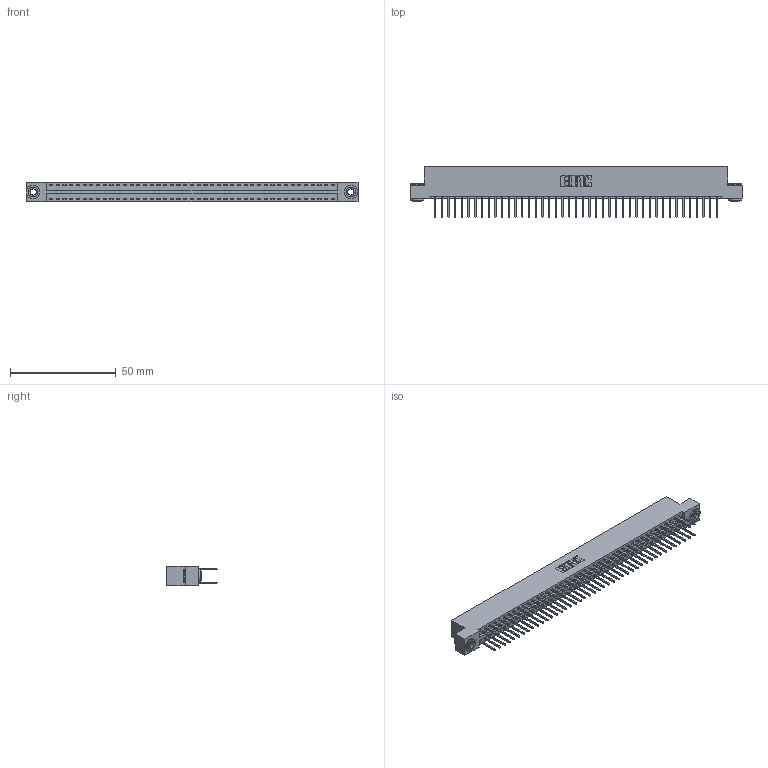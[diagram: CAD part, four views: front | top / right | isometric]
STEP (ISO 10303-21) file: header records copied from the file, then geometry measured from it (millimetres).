
FILE_DESCRIPTION (( 'STEP AP203' ), '1' );
FILE_NAME ('346-086-526-203.STEP', '2022-05-25T22:15:16', ( '' ), ( '' ), 'SwSTEP 2.0', 'SolidWorks 2020', '' );
FILE_SCHEMA (( 'CONFIG_CONTROL_DESIGN' ));
Length unit declared in the file: inch
Products named in the file (4): 345-292-001_345-293-126; 346 Part_Flush Mounting Lugs - 0.156 Dia-TH; 346-086-526-203; 345-250-002_345-250-002-102
Assembly tree (89 placements, depth 2):
  346-086-526-203
    346 Part_Flush Mounting Lugs - 0.156 Dia-TH
    345-292-001_345-293-126  x86
    345-250-002_345-250-002-102  x2
Bounding box: 157.1 x 24.13 x 9.4 mm (x, y, z)
Volume: 15469.2 mm3; surface area: 22159.1 mm2
Topology: 89 solids, 89 shells, 4646 faces, 13771 edges, 9062 vertices
Faces by surface type: plane 3110, cylinder 1528, cone 8
Entity records: 29012 total; most frequent: CARTESIAN_POINT 4761, ORIENTED_EDGE 4686, DIRECTION 4277, EDGE_CURVE 2343, LINE 2015, VECTOR 2015, VERTEX_POINT 1558, AXIS2_PLACEMENT_3D 1131
